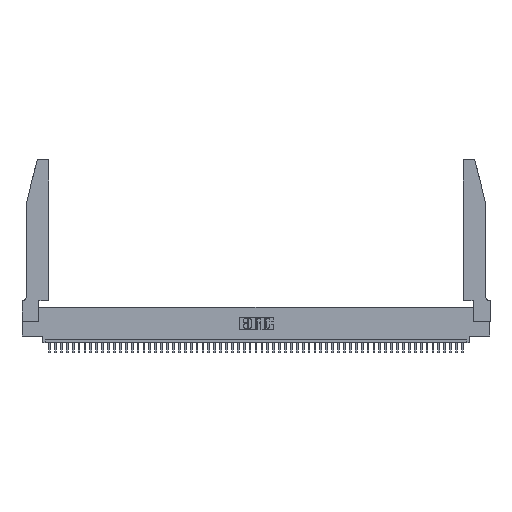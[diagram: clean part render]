
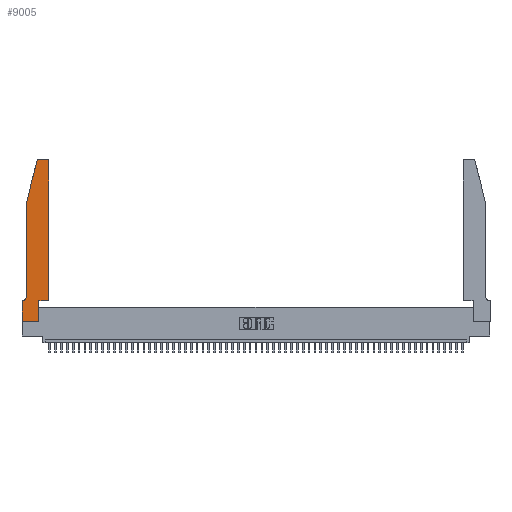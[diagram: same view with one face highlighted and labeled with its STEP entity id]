
A CAD part, top view. The second image highlights one B-rep face of the part: STEP entity #9005.
In plain terms, the highlighted planar face has unit normal (0, 0, 1).
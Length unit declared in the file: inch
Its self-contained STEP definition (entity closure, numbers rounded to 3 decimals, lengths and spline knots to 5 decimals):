
#301 = EDGE_CURVE ( 'NONE', #34338, #9859, #4396, .T. ) ;
#1783 = CARTESIAN_POINT ( 'NONE',  ( 0.2865, 0., 0.37 ) ) ;
#3197 = DIRECTION ( 'NONE',  ( -1., 0., 0. ) ) ;
#4396 = LINE ( 'NONE', #27137, #47801 ) ;
#4530 = CARTESIAN_POINT ( 'NONE',  ( 0.4505, 0.35, 0.37 ) ) ;
#4725 = VERTEX_POINT ( 'NONE', #11714 ) ;
#5195 = ORIENTED_EDGE ( 'NONE', *, *, #39259, .T. ) ;
#5390 = CARTESIAN_POINT ( 'NONE',  ( 0.284, 2.75, 0.37 ) ) ;
#5858 = EDGE_LOOP ( 'NONE', ( #6985, #35926, #36000, #47369, #5195, #26821, #38940, #13142, #15270, #28413, #33405, #34710 ) ) ;
#6192 = EDGE_CURVE ( 'NONE', #4725, #34338, #53472, .T. ) ;
#6318 = VERTEX_POINT ( 'NONE', #1783 ) ;
#6424 = DIRECTION ( 'NONE',  ( 0., -1., 0. ) ) ;
#6577 = CARTESIAN_POINT ( 'NONE',  ( 0.2865, 0.35, 0.37 ) ) ;
#6985 = ORIENTED_EDGE ( 'NONE', *, *, #301, .T. ) ;
#7109 = EDGE_CURVE ( 'NONE', #40939, #6318, #50108, .T. ) ;
#7860 = CARTESIAN_POINT ( 'NONE',  ( 0.0755, 2., 0.37 ) ) ;
#8148 = DIRECTION ( 'NONE',  ( -0.239, -0.971, 0. ) ) ;
#8258 = CARTESIAN_POINT ( 'NONE',  ( 0.0055, 0.35, 0.37 ) ) ;
#9005 = ADVANCED_FACE ( 'NONE', ( #48611 ), #43363, .T. ) ;
#9532 = CARTESIAN_POINT ( 'NONE',  ( 0., 0.35, 0.37 ) ) ;
#9859 = VERTEX_POINT ( 'NONE', #5390 ) ;
#10214 = DIRECTION ( 'NONE',  ( 0., 0., 1. ) ) ;
#11706 = DIRECTION ( 'NONE',  ( -1., 0., 0. ) ) ;
#11714 = CARTESIAN_POINT ( 'NONE',  ( 0.4505, 2.72, 0.37 ) ) ;
#11931 = VERTEX_POINT ( 'NONE', #29254 ) ;
#13142 = ORIENTED_EDGE ( 'NONE', *, *, #7109, .T. ) ;
#13198 = DIRECTION ( 'NONE',  ( 0., 0., 1. ) ) ;
#14081 = DIRECTION ( 'NONE',  ( 1., 0., 0. ) ) ;
#14640 = VERTEX_POINT ( 'NONE', #41328 ) ;
#15270 = ORIENTED_EDGE ( 'NONE', *, *, #47400, .T. ) ;
#15367 = VECTOR ( 'NONE', #52258, 39.37008 ) ;
#15815 = CARTESIAN_POINT ( 'NONE',  ( 0., 0.35, 0.37 ) ) ;
#16830 = VECTOR ( 'NONE', #3197, 39.37008 ) ;
#19419 = DIRECTION ( 'NONE',  ( 1., 0., 0. ) ) ;
#19856 = EDGE_CURVE ( 'NONE', #9859, #11931, #25304, .T. ) ;
#21334 = CARTESIAN_POINT ( 'NONE',  ( 0.284, 2.72, 0.37 ) ) ;
#21810 = EDGE_CURVE ( 'NONE', #22647, #40939, #45549, .T. ) ;
#21859 = LINE ( 'NONE', #31482, #15367 ) ;
#21969 = VECTOR ( 'NONE', #35942, 39.37008 ) ;
#22245 = DIRECTION ( 'NONE',  ( 0., 0., -1. ) ) ;
#22647 = VERTEX_POINT ( 'NONE', #15815 ) ;
#23108 = DIRECTION ( 'NONE',  ( 1., 0., 0. ) ) ;
#23531 = CARTESIAN_POINT ( 'NONE',  ( 0., 0., 0.37 ) ) ;
#23797 = VECTOR ( 'NONE', #14081, 39.37008 ) ;
#24723 = CIRCLE ( 'NONE', #51781, 0.07 ) ;
#24904 = LINE ( 'NONE', #32432, #54463 ) ;
#25304 = CIRCLE ( 'NONE', #49238, 0.03 ) ;
#26821 = ORIENTED_EDGE ( 'NONE', *, *, #38941, .T. ) ;
#26934 = CARTESIAN_POINT ( 'NONE',  ( 0.0755, 0.42, 0.37 ) ) ;
#27137 = CARTESIAN_POINT ( 'NONE',  ( 0.2605, 2.75, 0.37 ) ) ;
#28240 = AXIS2_PLACEMENT_3D ( 'NONE', #48096, #10214, #23108 ) ;
#28397 = CARTESIAN_POINT ( 'NONE',  ( 0.4505, 0.35, 0.37 ) ) ;
#28413 = ORIENTED_EDGE ( 'NONE', *, *, #52744, .T. ) ;
#28576 = CARTESIAN_POINT ( 'NONE',  ( 0.0755, 0.35, 0.37 ) ) ;
#29254 = CARTESIAN_POINT ( 'NONE',  ( 0.25487, 2.72718, 0.37 ) ) ;
#31482 = CARTESIAN_POINT ( 'NONE',  ( 0.4505, 0.35, 0.37 ) ) ;
#32298 = CARTESIAN_POINT ( 'NONE',  ( 0.0755, 2., 0.37 ) ) ;
#32432 = CARTESIAN_POINT ( 'NONE',  ( 0.0755, 2., 0.37 ) ) ;
#32567 = VECTOR ( 'NONE', #19419, 39.37008 ) ;
#32632 = EDGE_CURVE ( 'NONE', #53393, #36628, #40765, .T. ) ;
#33405 = ORIENTED_EDGE ( 'NONE', *, *, #48052, .T. ) ;
#33485 = CARTESIAN_POINT ( 'NONE',  ( 0.4205, 2.75, 0.37 ) ) ;
#34338 = VERTEX_POINT ( 'NONE', #33485 ) ;
#34556 = CARTESIAN_POINT ( 'NONE',  ( 0.0055, 0.42, 0.37 ) ) ;
#34710 = ORIENTED_EDGE ( 'NONE', *, *, #6192, .T. ) ;
#35926 = ORIENTED_EDGE ( 'NONE', *, *, #19856, .T. ) ;
#35942 = DIRECTION ( 'NONE',  ( 0., 1., 0. ) ) ;
#36000 = ORIENTED_EDGE ( 'NONE', *, *, #45332, .T. ) ;
#36628 = VERTEX_POINT ( 'NONE', #26934 ) ;
#36975 = VECTOR ( 'NONE', #6424, 39.37008 ) ;
#38438 = LINE ( 'NONE', #28397, #32567 ) ;
#38787 = DIRECTION ( 'NONE',  ( -1., 0., 0. ) ) ;
#38940 = ORIENTED_EDGE ( 'NONE', *, *, #21810, .T. ) ;
#38941 = EDGE_CURVE ( 'NONE', #46045, #22647, #43080, .T. ) ;
#39259 = EDGE_CURVE ( 'NONE', #36628, #46045, #24723, .T. ) ;
#39270 = CARTESIAN_POINT ( 'NONE',  ( 0., 0., 0.37 ) ) ;
#39500 = DIRECTION ( 'NONE',  ( 1., 0., 0. ) ) ;
#40765 = LINE ( 'NONE', #32298, #49294 ) ;
#40939 = VERTEX_POINT ( 'NONE', #45152 ) ;
#41328 = CARTESIAN_POINT ( 'NONE',  ( 0.2865, 0.35, 0.37 ) ) ;
#42491 = DIRECTION ( 'NONE',  ( 1., 0., 0. ) ) ;
#43080 = LINE ( 'NONE', #28576, #16830 ) ;
#43171 = DIRECTION ( 'NONE',  ( 0., 0., 1. ) ) ;
#43363 = PLANE ( 'NONE',  #51532 ) ;
#45152 = CARTESIAN_POINT ( 'NONE',  ( 0., 0., 0.37 ) ) ;
#45332 = EDGE_CURVE ( 'NONE', #11931, #53393, #24904, .T. ) ;
#45549 = LINE ( 'NONE', #23531, #36975 ) ;
#46045 = VERTEX_POINT ( 'NONE', #8258 ) ;
#46210 = VERTEX_POINT ( 'NONE', #4530 ) ;
#47369 = ORIENTED_EDGE ( 'NONE', *, *, #32632, .T. ) ;
#47400 = EDGE_CURVE ( 'NONE', #6318, #14640, #50303, .T. ) ;
#47801 = VECTOR ( 'NONE', #11706, 39.37008 ) ;
#48052 = EDGE_CURVE ( 'NONE', #46210, #4725, #21859, .T. ) ;
#48096 = CARTESIAN_POINT ( 'NONE',  ( 0.4205, 2.72, 0.37 ) ) ;
#48611 = FACE_OUTER_BOUND ( 'NONE', #5858, .T. ) ;
#49238 = AXIS2_PLACEMENT_3D ( 'NONE', #21334, #13198, #42491 ) ;
#49294 = VECTOR ( 'NONE', #53442, 39.37008 ) ;
#50108 = LINE ( 'NONE', #39270, #23797 ) ;
#50303 = LINE ( 'NONE', #6577, #21969 ) ;
#51532 = AXIS2_PLACEMENT_3D ( 'NONE', #9532, #43171, #39500 ) ;
#51781 = AXIS2_PLACEMENT_3D ( 'NONE', #34556, #22245, #38787 ) ;
#52258 = DIRECTION ( 'NONE',  ( 0., 1., 0. ) ) ;
#52744 = EDGE_CURVE ( 'NONE', #14640, #46210, #38438, .T. ) ;
#53393 = VERTEX_POINT ( 'NONE', #7860 ) ;
#53442 = DIRECTION ( 'NONE',  ( 0., -1., 0. ) ) ;
#53472 = CIRCLE ( 'NONE', #28240, 0.03 ) ;
#54463 = VECTOR ( 'NONE', #8148, 39.37008 ) ;
